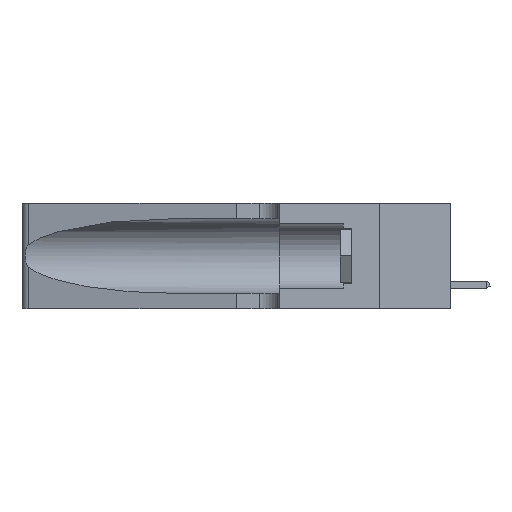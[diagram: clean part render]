
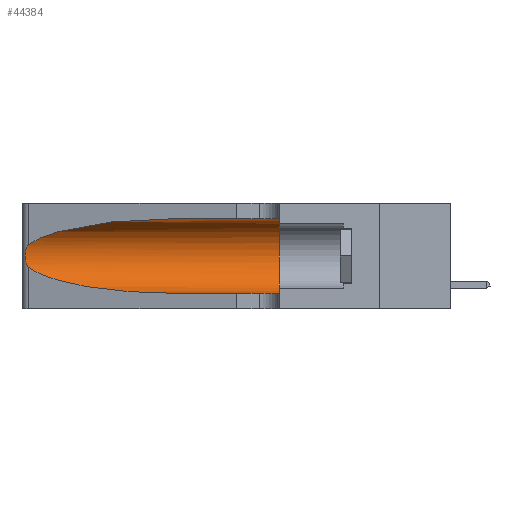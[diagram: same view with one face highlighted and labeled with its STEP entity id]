
A CAD part, left-side view. The second image highlights one B-rep face of the part: STEP entity #44384.
In plain terms, the highlighted cylindrical face has radius 3.308 mm (diameter 6.617 mm), a partial arc.
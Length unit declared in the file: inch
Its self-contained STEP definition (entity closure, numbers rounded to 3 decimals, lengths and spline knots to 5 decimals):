
#589 = CARTESIAN_POINT ( 'NONE',  ( 0.1305, 0.35, 0.31525 ) ) ;
#3065 = CARTESIAN_POINT ( 'NONE',  ( 0.1305, 1.61858, 0.05475 ) ) ;
#3226 = ORIENTED_EDGE ( 'NONE', *, *, #6643, .T. ) ;
#4176 = CYLINDRICAL_SURFACE ( 'NONE', #16563, 0.13025 ) ;
#5352 = CARTESIAN_POINT ( 'NONE',  ( 0.26075, 1.23896, 0.19203 ) ) ;
#5827 = CARTESIAN_POINT ( 'NONE',  ( 0.25487, 1.22718, 0.14631 ) ) ;
#6643 = EDGE_CURVE ( 'NONE', #43154, #36195, #43667, .T. ) ;
#6965 = LINE ( 'NONE', #25890, #37137 ) ;
#7029 = EDGE_CURVE ( 'NONE', #49457, #43154, #22282, .T. ) ;
#8083 = CARTESIAN_POINT ( 'NONE',  ( 0.25487, 1.22718, 0.14631 ) ) ;
#9177 = CARTESIAN_POINT ( 'NONE',  ( 0.25487, 1.22718, 0.22369 ) ) ;
#10060 = DIRECTION ( 'NONE',  ( 0., 1., 0. ) ) ;
#10319 = CIRCLE ( 'NONE', #11244, 0.13025 ) ;
#11244 = AXIS2_PLACEMENT_3D ( 'NONE', #33845, #10060, #22192 ) ;
#12139 = CARTESIAN_POINT ( 'NONE',  ( 0.18966, 0.96281, 0.31525 ) ) ;
#12724 = EDGE_CURVE ( 'NONE', #36195, #41004, #46846, .T. ) ;
#14695 = CARTESIAN_POINT ( 'NONE',  ( 0.25555, 1.22993, 0.14849 ) ) ;
#14999 = ORIENTED_EDGE ( 'NONE', *, *, #7029, .T. ) ;
#15378 = FACE_OUTER_BOUND ( 'NONE', #28756, .T. ) ;
#16563 = AXIS2_PLACEMENT_3D ( 'NONE', #17348, #33712, #21687 ) ;
#16598 = CARTESIAN_POINT ( 'NONE',  ( 0.25555, 1.22994, 0.2215 ) ) ;
#17348 = CARTESIAN_POINT ( 'NONE',  ( 0.1305, 1.61858, 0.185 ) ) ;
#18394 = EDGE_CURVE ( 'NONE', #38486, #28450, #10319, .T. ) ;
#19834 = ORIENTED_EDGE ( 'NONE', *, *, #18394, .F. ) ;
#20649 = ORIENTED_EDGE ( 'NONE', *, *, #12724, .T. ) ;
#21687 = DIRECTION ( 'NONE',  ( 0., 0., -1. ) ) ;
#22192 = DIRECTION ( 'NONE',  ( 0., 0., 1. ) ) ;
#22282 =( BOUNDED_CURVE ( )  B_SPLINE_CURVE ( 3, ( #24371, #12139, #40560, #9177 ),
 .UNSPECIFIED., .F., .F. ) 
 B_SPLINE_CURVE_WITH_KNOTS ( ( 4, 4 ),
 ( 1.5708, 2.84003 ),
 .UNSPECIFIED. ) 
 CURVE ( )  GEOMETRIC_REPRESENTATION_ITEM ( )  RATIONAL_B_SPLINE_CURVE ( ( 1., 0.87, 0.87, 1. ) ) 
 REPRESENTATION_ITEM ( '' )  );
#22826 = CARTESIAN_POINT ( 'NONE',  ( 0.25789, 1.23486, 0.15765 ) ) ;
#24049 = CARTESIAN_POINT ( 'NONE',  ( 0.1305, 0.35, 0.05475 ) ) ;
#24371 = CARTESIAN_POINT ( 'NONE',  ( 0.1305, 0.72297, 0.31525 ) ) ;
#25890 = CARTESIAN_POINT ( 'NONE',  ( 0.1305, 1.61858, 0.31525 ) ) ;
#26548 = LINE ( 'NONE', #3065, #44993 ) ;
#28450 = VERTEX_POINT ( 'NONE', #24049 ) ;
#28756 = EDGE_LOOP ( 'NONE', ( #14999, #3226, #20649, #37685, #19834, #38565 ) ) ;
#28960 = CARTESIAN_POINT ( 'NONE',  ( 0.25787, 1.23484, 0.2124 ) ) ;
#28964 = CARTESIAN_POINT ( 'NONE',  ( 0.25487, 1.22718, 0.22369 ) ) ;
#30369 = CARTESIAN_POINT ( 'NONE',  ( 0.26017, 1.23833, 0.17102 ) ) ;
#30495 = CARTESIAN_POINT ( 'NONE',  ( 0.1305, 0.72297, 0.05475 ) ) ;
#32933 = CARTESIAN_POINT ( 'NONE',  ( 0.26075, 1.23896, 0.178 ) ) ;
#33712 = DIRECTION ( 'NONE',  ( 0., -1., 0. ) ) ;
#33735 = EDGE_CURVE ( 'NONE', #49457, #38486, #6965, .T. ) ;
#33845 = CARTESIAN_POINT ( 'NONE',  ( 0.1305, 0.35, 0.185 ) ) ;
#34288 = CARTESIAN_POINT ( 'NONE',  ( 0.18966, 0.96281, 0.05475 ) ) ;
#34328 = DIRECTION ( 'NONE',  ( 0., -1., 0. ) ) ;
#35665 = CARTESIAN_POINT ( 'NONE',  ( 0.1305, 0.72297, 0.05475 ) ) ;
#36195 = VERTEX_POINT ( 'NONE', #42373 ) ;
#37072 = CARTESIAN_POINT ( 'NONE',  ( 0.25854, 1.2359, 0.20912 ) ) ;
#37113 = CARTESIAN_POINT ( 'NONE',  ( 0.1305, 0.72297, 0.31525 ) ) ;
#37137 = VECTOR ( 'NONE', #34328, 39.37008 ) ;
#37428 = CARTESIAN_POINT ( 'NONE',  ( 0.25639, 1.23184, 0.21858 ) ) ;
#37685 = ORIENTED_EDGE ( 'NONE', *, *, #44031, .T. ) ;
#38486 = VERTEX_POINT ( 'NONE', #589 ) ;
#38565 = ORIENTED_EDGE ( 'NONE', *, *, #33735, .F. ) ;
#40560 = CARTESIAN_POINT ( 'NONE',  ( 0.2373, 1.15595, 0.28018 ) ) ;
#41004 = VERTEX_POINT ( 'NONE', #35665 ) ;
#41553 = CARTESIAN_POINT ( 'NONE',  ( 0.26018, 1.23835, 0.19895 ) ) ;
#42373 = CARTESIAN_POINT ( 'NONE',  ( 0.25487, 1.22718, 0.14631 ) ) ;
#43154 = VERTEX_POINT ( 'NONE', #28964 ) ;
#43667 = B_SPLINE_CURVE_WITH_KNOTS ( 'NONE', 3,
 ( #46301, #16598, #37428, #28960, #37072, #41553, #5352, #32933, #30369, #49631, #22826, #50325, #14695, #8083 ),
 .UNSPECIFIED., .F., .F.,
 ( 4, 2, 2, 2, 2, 2, 4 ),
 ( 0., 0.00027, 0.00053, 0.00107, 0.0016, 0.00187, 0.00214 ),
 .UNSPECIFIED. ) ;
#44031 = EDGE_CURVE ( 'NONE', #41004, #28450, #26548, .T. ) ;
#44384 = ADVANCED_FACE ( 'NONE', ( #15378 ), #4176, .F. ) ;
#44993 = VECTOR ( 'NONE', #47653, 39.37008 ) ;
#46301 = CARTESIAN_POINT ( 'NONE',  ( 0.25487, 1.22718, 0.22369 ) ) ;
#46520 = CARTESIAN_POINT ( 'NONE',  ( 0.2373, 1.15595, 0.08982 ) ) ;
#46846 =( BOUNDED_CURVE ( )  B_SPLINE_CURVE ( 3, ( #5827, #46520, #34288, #30495 ),
 .UNSPECIFIED., .F., .F. ) 
 B_SPLINE_CURVE_WITH_KNOTS ( ( 4, 4 ),
 ( 3.44316, 4.71239 ),
 .UNSPECIFIED. ) 
 CURVE ( )  GEOMETRIC_REPRESENTATION_ITEM ( )  RATIONAL_B_SPLINE_CURVE ( ( 1., 0.87, 0.87, 1. ) ) 
 REPRESENTATION_ITEM ( '' )  );
#47653 = DIRECTION ( 'NONE',  ( 0., -1., 0. ) ) ;
#49457 = VERTEX_POINT ( 'NONE', #37113 ) ;
#49631 = CARTESIAN_POINT ( 'NONE',  ( 0.25856, 1.23593, 0.16098 ) ) ;
#50325 = CARTESIAN_POINT ( 'NONE',  ( 0.25639, 1.23186, 0.15144 ) ) ;
